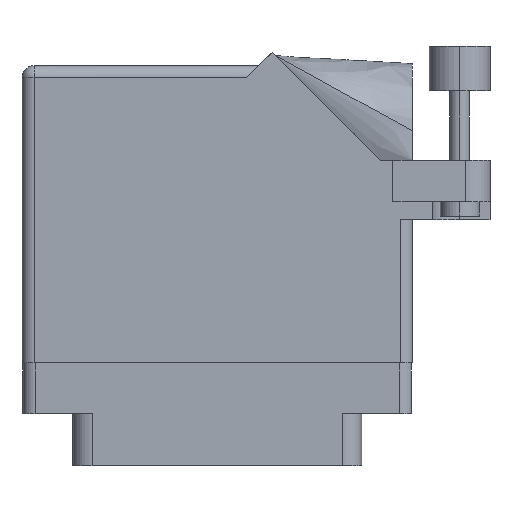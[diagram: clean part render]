
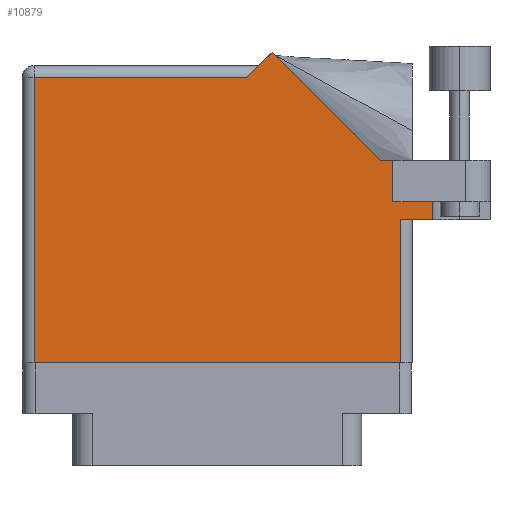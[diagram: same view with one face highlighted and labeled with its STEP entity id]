
A CAD part, front view. The second image highlights one B-rep face of the part: STEP entity #10879.
In plain terms, the highlighted face is planar.
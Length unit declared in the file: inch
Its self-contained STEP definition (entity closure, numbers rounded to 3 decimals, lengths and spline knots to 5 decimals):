
#46 = ORIENTED_EDGE ( 'NONE', *, *, #18542, .T. ) ;
#695 = ORIENTED_EDGE ( 'NONE', *, *, #16603, .T. ) ;
#844 = DIRECTION ( 'NONE',  ( -0.707, 0.707, 0. ) ) ;
#1061 = CARTESIAN_POINT ( 'NONE',  ( 1.28771, 1.60071, 0. ) ) ;
#1246 = DIRECTION ( 'NONE',  ( 0., 1., 0. ) ) ;
#1504 = CARTESIAN_POINT ( 'NONE',  ( 1.91, 0.831, 0. ) ) ;
#1525 = ORIENTED_EDGE ( 'NONE', *, *, #12270, .T. ) ;
#2574 = LINE ( 'NONE', #4030, #23541 ) ;
#3756 = VERTEX_POINT ( 'NONE', #9834 ) ;
#4030 = CARTESIAN_POINT ( 'NONE',  ( 1.217, 1.53, 0. ) ) ;
#4751 = DIRECTION ( 'NONE',  ( 0., -1., 0. ) ) ;
#5821 = VERTEX_POINT ( 'NONE', #33937 ) ;
#6738 = EDGE_CURVE ( 'NONE', #26226, #28350, #22732, .T. ) ;
#7833 = LINE ( 'NONE', #29807, #20275 ) ;
#8039 = CARTESIAN_POINT ( 'NONE',  ( 1.155, 1.468, 0. ) ) ;
#8309 = FACE_OUTER_BOUND ( 'NONE', #10595, .T. ) ;
#8344 = VECTOR ( 'NONE', #844, 39.37008 ) ;
#8391 = VECTOR ( 'NONE', #18192, 39.37008 ) ;
#8399 = VECTOR ( 'NONE', #20498, 39.37008 ) ;
#8745 = CARTESIAN_POINT ( 'NONE',  ( 0.062, 1.468, 0. ) ) ;
#9135 = VECTOR ( 'NONE', #17328, 39.37008 ) ;
#9834 = CARTESIAN_POINT ( 'NONE',  ( 2.1115, 0.831, 0. ) ) ;
#10078 = CARTESIAN_POINT ( 'NONE',  ( 1.91, 0.831, 0. ) ) ;
#10279 = LINE ( 'NONE', #12019, #8391 ) ;
#10302 = VECTOR ( 'NONE', #1246, 39.37008 ) ;
#10514 = EDGE_CURVE ( 'NONE', #34631, #15913, #34094, .T. ) ;
#10595 = EDGE_LOOP ( 'NONE', ( #17962, #1525, #22063, #30219, #26251, #38032, #46, #11678, #20736, #25024, #695 ) ) ;
#10879 = ADVANCED_FACE ( 'NONE', ( #8309 ), #20539, .F. ) ;
#10965 = VERTEX_POINT ( 'NONE', #8745 ) ;
#10970 = CARTESIAN_POINT ( 'NONE',  ( 1.948, 0., 0. ) ) ;
#11279 = CARTESIAN_POINT ( 'NONE',  ( 2.41, 1.044, 0. ) ) ;
#11675 = DIRECTION ( 'NONE',  ( 1., 0., 0. ) ) ;
#11678 = ORIENTED_EDGE ( 'NONE', *, *, #10514, .T. ) ;
#12019 = CARTESIAN_POINT ( 'NONE',  ( 0., 1.468, 0. ) ) ;
#12258 = EDGE_CURVE ( 'NONE', #26226, #3756, #23933, .T. ) ;
#12270 = EDGE_CURVE ( 'NONE', #32972, #38231, #12449, .T. ) ;
#12449 = LINE ( 'NONE', #34645, #27688 ) ;
#13112 = CARTESIAN_POINT ( 'NONE',  ( 0.062, 0., 0. ) ) ;
#15913 = VERTEX_POINT ( 'NONE', #1061 ) ;
#16339 = DIRECTION ( 'NONE',  ( -0.707, -0.707, 0. ) ) ;
#16603 = EDGE_CURVE ( 'NONE', #10965, #28005, #37808, .T. ) ;
#16681 = DIRECTION ( 'NONE',  ( 0., 1., 0. ) ) ;
#17240 = DIRECTION ( 'NONE',  ( 0., 0., -1. ) ) ;
#17328 = DIRECTION ( 'NONE',  ( -1., 0., 0. ) ) ;
#17335 = LINE ( 'NONE', #11279, #9135 ) ;
#17795 = VECTOR ( 'NONE', #28462, 39.37008 ) ;
#17962 = ORIENTED_EDGE ( 'NONE', *, *, #32421, .T. ) ;
#18192 = DIRECTION ( 'NONE',  ( -1., 0., 0. ) ) ;
#18542 = EDGE_CURVE ( 'NONE', #28350, #34631, #17335, .T. ) ;
#19413 = LINE ( 'NONE', #38693, #8399 ) ;
#20019 = CARTESIAN_POINT ( 'NONE',  ( 0., 1.53, 0. ) ) ;
#20275 = VECTOR ( 'NONE', #11675, 39.37008 ) ;
#20498 = DIRECTION ( 'NONE',  ( 1., 0., 0. ) ) ;
#20539 = PLANE ( 'NONE',  #37346 ) ;
#20736 = ORIENTED_EDGE ( 'NONE', *, *, #32698, .T. ) ;
#20835 = CARTESIAN_POINT ( 'NONE',  ( 1.84442, 1.044, 0. ) ) ;
#20846 = CARTESIAN_POINT ( 'NONE',  ( 1.91, 1.044, 0. ) ) ;
#20991 = EDGE_CURVE ( 'NONE', #25944, #10965, #10279, .T. ) ;
#21880 = VECTOR ( 'NONE', #28015, 39.37008 ) ;
#22063 = ORIENTED_EDGE ( 'NONE', *, *, #30937, .T. ) ;
#22732 = LINE ( 'NONE', #1504, #10302 ) ;
#23541 = VECTOR ( 'NONE', #16339, 39.37008 ) ;
#23933 = LINE ( 'NONE', #10078, #17795 ) ;
#25024 = ORIENTED_EDGE ( 'NONE', *, *, #20991, .T. ) ;
#25944 = VERTEX_POINT ( 'NONE', #8039 ) ;
#26226 = VERTEX_POINT ( 'NONE', #32462 ) ;
#26251 = ORIENTED_EDGE ( 'NONE', *, *, #12258, .F. ) ;
#27688 = VECTOR ( 'NONE', #16681, 39.37008 ) ;
#28005 = VERTEX_POINT ( 'NONE', #13112 ) ;
#28015 = DIRECTION ( 'NONE',  ( 0., -1., 0. ) ) ;
#28350 = VERTEX_POINT ( 'NONE', #20846 ) ;
#28462 = DIRECTION ( 'NONE',  ( 1., 0., 0. ) ) ;
#29807 = CARTESIAN_POINT ( 'NONE',  ( 0., 0., 0. ) ) ;
#30219 = ORIENTED_EDGE ( 'NONE', *, *, #39092, .F. ) ;
#30916 = LINE ( 'NONE', #37605, #21880 ) ;
#30937 = EDGE_CURVE ( 'NONE', #38231, #5821, #19413, .T. ) ;
#32421 = EDGE_CURVE ( 'NONE', #28005, #32972, #7833, .T. ) ;
#32462 = CARTESIAN_POINT ( 'NONE',  ( 1.91, 0.831, 0. ) ) ;
#32521 = CARTESIAN_POINT ( 'NONE',  ( 0.062, 0., 0. ) ) ;
#32698 = EDGE_CURVE ( 'NONE', #15913, #25944, #2574, .T. ) ;
#32972 = VERTEX_POINT ( 'NONE', #10970 ) ;
#33577 = VECTOR ( 'NONE', #4751, 39.37008 ) ;
#33937 = CARTESIAN_POINT ( 'NONE',  ( 2.1115, 0.737, 0. ) ) ;
#34094 = LINE ( 'NONE', #37361, #8344 ) ;
#34631 = VERTEX_POINT ( 'NONE', #20835 ) ;
#34645 = CARTESIAN_POINT ( 'NONE',  ( 1.948, 0.737, 0. ) ) ;
#36741 = CARTESIAN_POINT ( 'NONE',  ( 1.948, 0.737, 0. ) ) ;
#37346 = AXIS2_PLACEMENT_3D ( 'NONE', #20019, #17240, #38477 ) ;
#37361 = CARTESIAN_POINT ( 'NONE',  ( 1.84442, 1.044, 0. ) ) ;
#37605 = CARTESIAN_POINT ( 'NONE',  ( 2.1115, 1.16177, 0. ) ) ;
#37808 = LINE ( 'NONE', #32521, #33577 ) ;
#38032 = ORIENTED_EDGE ( 'NONE', *, *, #6738, .T. ) ;
#38231 = VERTEX_POINT ( 'NONE', #36741 ) ;
#38477 = DIRECTION ( 'NONE',  ( -1., 0., 0. ) ) ;
#38693 = CARTESIAN_POINT ( 'NONE',  ( 2.01, 0.737, 0. ) ) ;
#39092 = EDGE_CURVE ( 'NONE', #3756, #5821, #30916, .T. ) ;
